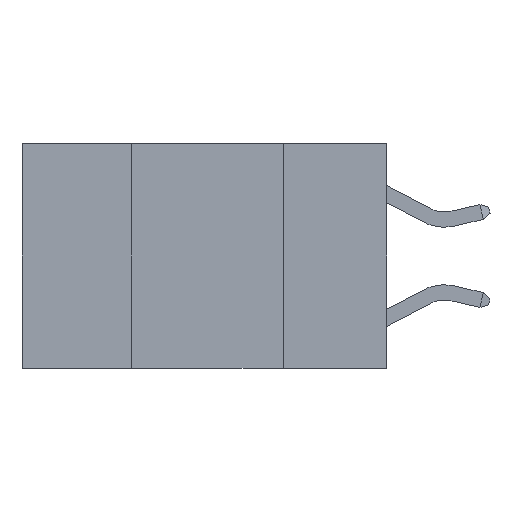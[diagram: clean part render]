
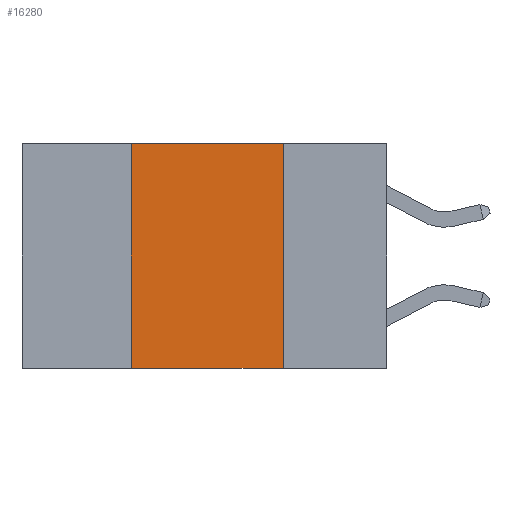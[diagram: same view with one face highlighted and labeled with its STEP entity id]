
A CAD part, left-side view. The second image highlights one B-rep face of the part: STEP entity #16280.
In plain terms, the highlighted planar face has unit normal (-1, 0, 0).
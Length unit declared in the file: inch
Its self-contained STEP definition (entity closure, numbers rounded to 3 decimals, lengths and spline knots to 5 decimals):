
#350 = VECTOR ( 'NONE', #23501, 39.37008 ) ;
#645 = VERTEX_POINT ( 'NONE', #6423 ) ;
#1238 = AXIS2_PLACEMENT_3D ( 'NONE', #8522, #26062, #6840 ) ;
#1278 = VERTEX_POINT ( 'NONE', #7286 ) ;
#1477 = VERTEX_POINT ( 'NONE', #17744 ) ;
#2247 = LINE ( 'NONE', #16994, #18320 ) ;
#2350 = FACE_OUTER_BOUND ( 'NONE', #13270, .T. ) ;
#2794 = DIRECTION ( 'NONE',  ( 0., 0., 1. ) ) ;
#3427 = VERTEX_POINT ( 'NONE', #3915 ) ;
#3915 = CARTESIAN_POINT ( 'NONE',  ( 0., 0.42, 0. ) ) ;
#4168 = EDGE_CURVE ( 'NONE', #1278, #645, #15391, .T. ) ;
#4561 = CARTESIAN_POINT ( 'NONE',  ( 0., 0.17, 0. ) ) ;
#4836 = DIRECTION ( 'NONE',  ( 0., 0., -1. ) ) ;
#4901 = LINE ( 'NONE', #13477, #11592 ) ;
#5395 = ORIENTED_EDGE ( 'NONE', *, *, #4168, .F. ) ;
#6423 = CARTESIAN_POINT ( 'NONE',  ( 0., 0.17, -0.37 ) ) ;
#6840 = DIRECTION ( 'NONE',  ( 0., 0., -1. ) ) ;
#7286 = CARTESIAN_POINT ( 'NONE',  ( 0., 0.17, 0. ) ) ;
#8522 = CARTESIAN_POINT ( 'NONE',  ( 0., 0.6, 0. ) ) ;
#10878 = CARTESIAN_POINT ( 'NONE',  ( 0., 0.6, 0. ) ) ;
#11592 = VECTOR ( 'NONE', #2794, 39.37008 ) ;
#13270 = EDGE_LOOP ( 'NONE', ( #5395, #21552, #13959, #23605 ) ) ;
#13477 = CARTESIAN_POINT ( 'NONE',  ( 0., 0.42, 0. ) ) ;
#13959 = ORIENTED_EDGE ( 'NONE', *, *, #19283, .F. ) ;
#15391 = LINE ( 'NONE', #4561, #16102 ) ;
#16102 = VECTOR ( 'NONE', #4836, 39.37008 ) ;
#16280 = ADVANCED_FACE ( 'NONE', ( #2350 ), #25774, .F. ) ;
#16822 = EDGE_CURVE ( 'NONE', #3427, #1278, #25878, .T. ) ;
#16994 = CARTESIAN_POINT ( 'NONE',  ( 0., 0.6, -0.37 ) ) ;
#17744 = CARTESIAN_POINT ( 'NONE',  ( 0., 0.42, -0.37 ) ) ;
#18320 = VECTOR ( 'NONE', #21107, 39.37008 ) ;
#19091 = EDGE_CURVE ( 'NONE', #1477, #645, #2247, .T. ) ;
#19283 = EDGE_CURVE ( 'NONE', #1477, #3427, #4901, .T. ) ;
#21107 = DIRECTION ( 'NONE',  ( 0., -1., 0. ) ) ;
#21552 = ORIENTED_EDGE ( 'NONE', *, *, #16822, .F. ) ;
#23501 = DIRECTION ( 'NONE',  ( 0., -1., 0. ) ) ;
#23605 = ORIENTED_EDGE ( 'NONE', *, *, #19091, .T. ) ;
#25774 = PLANE ( 'NONE',  #1238 ) ;
#25878 = LINE ( 'NONE', #10878, #350 ) ;
#26062 = DIRECTION ( 'NONE',  ( 1., 0., 0. ) ) ;
